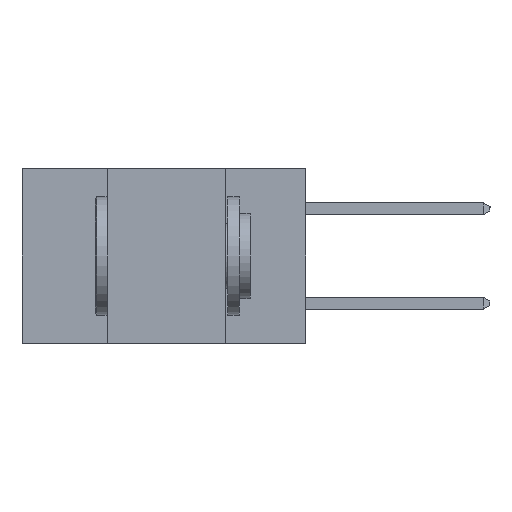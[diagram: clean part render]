
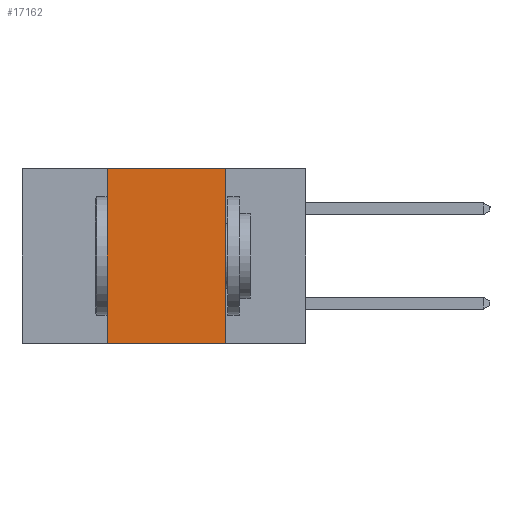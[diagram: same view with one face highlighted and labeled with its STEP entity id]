
A CAD part, left-side view. The second image highlights one B-rep face of the part: STEP entity #17162.
In plain terms, the highlighted planar face has unit normal (-1, 0, 0).
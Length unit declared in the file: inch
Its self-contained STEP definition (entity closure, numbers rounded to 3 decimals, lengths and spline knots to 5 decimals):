
#497 = DIRECTION ( 'NONE',  ( 0., -1., 0. ) ) ;
#982 = VERTEX_POINT ( 'NONE', #15440 ) ;
#1440 = EDGE_LOOP ( 'NONE', ( #4411, #17999, #16303, #13954 ) ) ;
#2983 = CARTESIAN_POINT ( 'NONE',  ( 0., 0.17, 0. ) ) ;
#4411 = ORIENTED_EDGE ( 'NONE', *, *, #13147, .F. ) ;
#4644 = VERTEX_POINT ( 'NONE', #2983 ) ;
#5650 = EDGE_CURVE ( 'NONE', #14375, #4644, #7476, .T. ) ;
#6579 = VECTOR ( 'NONE', #7897, 39.37008 ) ;
#6838 = DIRECTION ( 'NONE',  ( 0., 0., -1. ) ) ;
#7286 = DIRECTION ( 'NONE',  ( 0., 0., -1. ) ) ;
#7476 = LINE ( 'NONE', #12880, #13593 ) ;
#7635 = CARTESIAN_POINT ( 'NONE',  ( 0., 0.6, 0. ) ) ;
#7664 = LINE ( 'NONE', #13748, #6579 ) ;
#7897 = DIRECTION ( 'NONE',  ( 0., -1., 0. ) ) ;
#8629 = CARTESIAN_POINT ( 'NONE',  ( 0., 0.42, -0.37 ) ) ;
#9026 = AXIS2_PLACEMENT_3D ( 'NONE', #7635, #22047, #7286 ) ;
#10801 = FACE_OUTER_BOUND ( 'NONE', #1440, .T. ) ;
#12201 = VECTOR ( 'NONE', #15552, 39.37008 ) ;
#12267 = LINE ( 'NONE', #8629, #12201 ) ;
#12575 = CARTESIAN_POINT ( 'NONE',  ( 0., 0.17, -0.37 ) ) ;
#12880 = CARTESIAN_POINT ( 'NONE',  ( 0., 0.6, 0. ) ) ;
#13147 = EDGE_CURVE ( 'NONE', #4644, #19463, #14459, .T. ) ;
#13593 = VECTOR ( 'NONE', #497, 39.37008 ) ;
#13748 = CARTESIAN_POINT ( 'NONE',  ( 0., 0.6, -0.37 ) ) ;
#13954 = ORIENTED_EDGE ( 'NONE', *, *, #20041, .T. ) ;
#14375 = VERTEX_POINT ( 'NONE', #15536 ) ;
#14459 = LINE ( 'NONE', #12575, #16481 ) ;
#15440 = CARTESIAN_POINT ( 'NONE',  ( 0., 0.42, -0.37 ) ) ;
#15536 = CARTESIAN_POINT ( 'NONE',  ( 0., 0.42, 0. ) ) ;
#15552 = DIRECTION ( 'NONE',  ( 0., 0., 1. ) ) ;
#16303 = ORIENTED_EDGE ( 'NONE', *, *, #19661, .F. ) ;
#16481 = VECTOR ( 'NONE', #6838, 39.37008 ) ;
#16543 = PLANE ( 'NONE',  #9026 ) ;
#17162 = ADVANCED_FACE ( 'NONE', ( #10801 ), #16543, .F. ) ;
#17999 = ORIENTED_EDGE ( 'NONE', *, *, #5650, .F. ) ;
#19463 = VERTEX_POINT ( 'NONE', #19649 ) ;
#19649 = CARTESIAN_POINT ( 'NONE',  ( 0., 0.17, -0.37 ) ) ;
#19661 = EDGE_CURVE ( 'NONE', #982, #14375, #12267, .T. ) ;
#20041 = EDGE_CURVE ( 'NONE', #982, #19463, #7664, .T. ) ;
#22047 = DIRECTION ( 'NONE',  ( 1., 0., 0. ) ) ;
